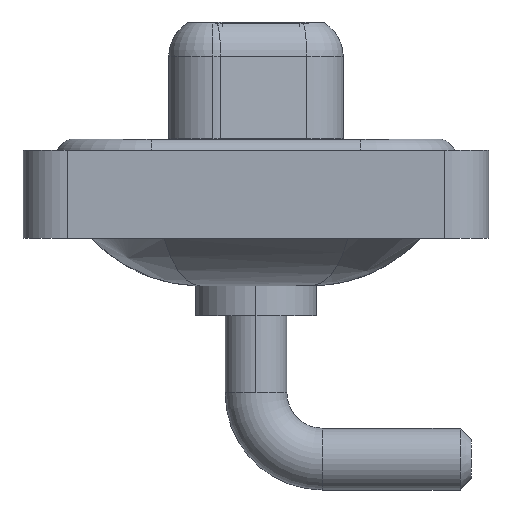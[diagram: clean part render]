
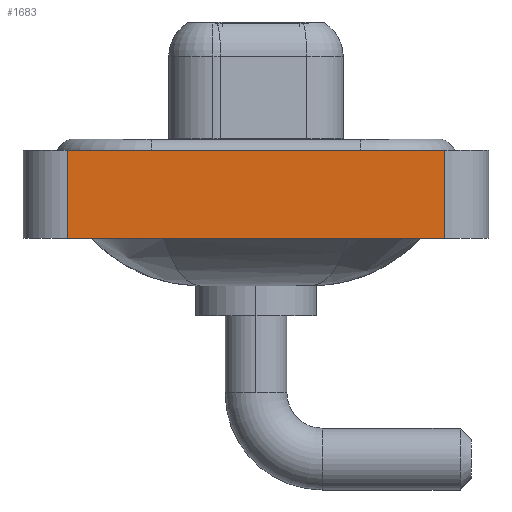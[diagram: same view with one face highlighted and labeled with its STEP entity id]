
A CAD part, left-side view. The second image highlights one B-rep face of the part: STEP entity #1683.
In plain terms, the highlighted planar face has unit normal (-1, 0, 0).
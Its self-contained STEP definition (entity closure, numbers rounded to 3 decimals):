
#96 = PLANE ( 'NONE',  #11218 ) ;
#145 = EDGE_CURVE ( 'NONE', #4362, #11150, #8270, .T. ) ;
#247 = VECTOR ( 'NONE', #3857, 1000. ) ;
#1002 = CARTESIAN_POINT ( 'NONE',  ( -7.3, 8.55, -3.6 ) ) ;
#1189 = EDGE_CURVE ( 'NONE', #11205, #11150, #15242, .T. ) ;
#1493 = CARTESIAN_POINT ( 'NONE',  ( -7.3, -8.55, 0.4 ) ) ;
#1683 = ADVANCED_FACE ( 'NONE', ( #7324 ), #96, .T. ) ;
#2380 = DIRECTION ( 'NONE',  ( 0., 0., 1. ) ) ;
#2431 = CARTESIAN_POINT ( 'NONE',  ( -7.3, -8.55, -3.6 ) ) ;
#3479 = CARTESIAN_POINT ( 'NONE',  ( -7.3, -8.55, -3.6 ) ) ;
#3535 = VECTOR ( 'NONE', #4759, 1000. ) ;
#3809 = CARTESIAN_POINT ( 'NONE',  ( -7.3, 8.55, -3.6 ) ) ;
#3857 = DIRECTION ( 'NONE',  ( 0., 0., 1. ) ) ;
#4362 = VERTEX_POINT ( 'NONE', #7182 ) ;
#4671 = DIRECTION ( 'NONE',  ( 0., 0., 1. ) ) ;
#4759 = DIRECTION ( 'NONE',  ( 0., -1., 0. ) ) ;
#5648 = ORIENTED_EDGE ( 'NONE', *, *, #1189, .T. ) ;
#6264 = ORIENTED_EDGE ( 'NONE', *, *, #15924, .T. ) ;
#6713 = CARTESIAN_POINT ( 'NONE',  ( -7.3, -8.55, -3.6 ) ) ;
#7055 = VERTEX_POINT ( 'NONE', #1002 ) ;
#7182 = CARTESIAN_POINT ( 'NONE',  ( -7.3, 8.55, 0.4 ) ) ;
#7324 = FACE_OUTER_BOUND ( 'NONE', #13335, .T. ) ;
#7491 = LINE ( 'NONE', #3479, #3535 ) ;
#7664 = ORIENTED_EDGE ( 'NONE', *, *, #15349, .F. ) ;
#8270 = LINE ( 'NONE', #13211, #14608 ) ;
#10208 = VECTOR ( 'NONE', #2380, 1000. ) ;
#10324 = CARTESIAN_POINT ( 'NONE',  ( -7.3, -8.55, -3.6 ) ) ;
#11037 = DIRECTION ( 'NONE',  ( -1., 0., 0. ) ) ;
#11150 = VERTEX_POINT ( 'NONE', #1493 ) ;
#11205 = VERTEX_POINT ( 'NONE', #6713 ) ;
#11218 = AXIS2_PLACEMENT_3D ( 'NONE', #2431, #11037, #4671 ) ;
#13211 = CARTESIAN_POINT ( 'NONE',  ( -7.3, -8.55, 0.4 ) ) ;
#13335 = EDGE_LOOP ( 'NONE', ( #5648, #13611, #7664, #6264 ) ) ;
#13495 = LINE ( 'NONE', #3809, #10208 ) ;
#13611 = ORIENTED_EDGE ( 'NONE', *, *, #145, .F. ) ;
#14409 = DIRECTION ( 'NONE',  ( 0., -1., 0. ) ) ;
#14608 = VECTOR ( 'NONE', #14409, 1000. ) ;
#15242 = LINE ( 'NONE', #10324, #247 ) ;
#15349 = EDGE_CURVE ( 'NONE', #7055, #4362, #13495, .T. ) ;
#15924 = EDGE_CURVE ( 'NONE', #7055, #11205, #7491, .T. ) ;
